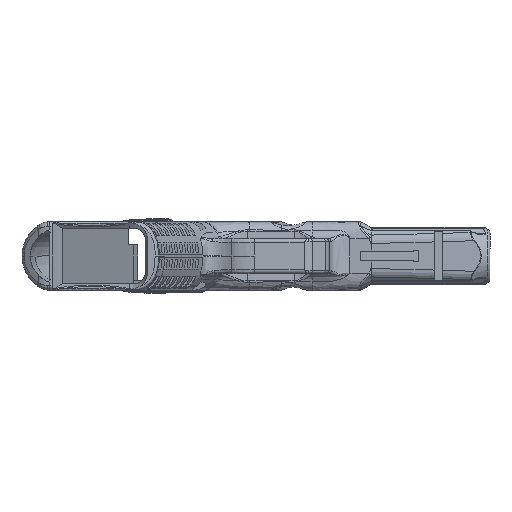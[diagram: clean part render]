
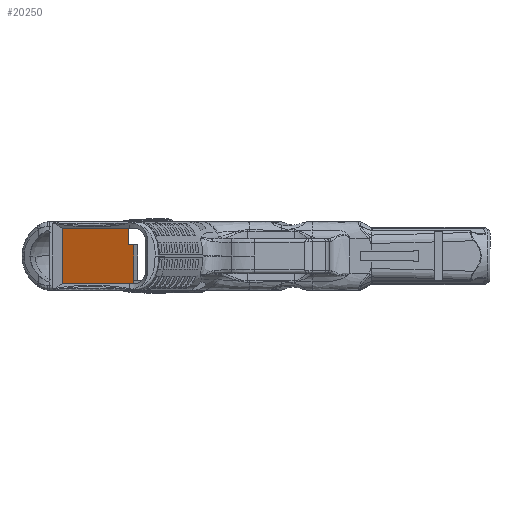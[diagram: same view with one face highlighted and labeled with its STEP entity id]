
A CAD part, front view. The second image highlights one B-rep face of the part: STEP entity #20250.
In plain terms, the highlighted planar face has unit normal (0.95, -0.311, 0).
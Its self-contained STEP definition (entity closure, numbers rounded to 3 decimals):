
#580=PLANE('',#21538);
#2908=FACE_OUTER_BOUND('',#4125,.T.);
#4125=EDGE_LOOP('',(#14632,#14633,#14634,#14635,#14636,#14637,#14638,#14639,
#14640,#14641,#14642));
#5301=LINE('',#34542,#6523);
#5313=LINE('',#35303,#6535);
#5354=LINE('',#42689,#6576);
#5384=LINE('',#45547,#6606);
#5385=LINE('',#45549,#6607);
#5386=LINE('',#45551,#6608);
#5387=LINE('',#45553,#6609);
#5388=LINE('',#45555,#6610);
#5389=LINE('',#45557,#6611);
#5390=LINE('',#45559,#6612);
#5391=LINE('',#45560,#6613);
#6523=VECTOR('',#23052,10.);
#6535=VECTOR('',#23108,10.);
#6576=VECTOR('',#23311,10.);
#6606=VECTOR('',#23455,1.);
#6607=VECTOR('',#23456,10.);
#6608=VECTOR('',#23457,1.);
#6609=VECTOR('',#23458,1.);
#6610=VECTOR('',#23459,1.);
#6611=VECTOR('',#23460,1.);
#6612=VECTOR('',#23461,1.);
#6613=VECTOR('',#23462,1.);
#8376=VERTEX_POINT('',#34539);
#8377=VERTEX_POINT('',#34541);
#8403=VERTEX_POINT('',#35300);
#8404=VERTEX_POINT('',#35302);
#8618=VERTEX_POINT('',#45546);
#8619=VERTEX_POINT('',#45548);
#8620=VERTEX_POINT('',#45550);
#8621=VERTEX_POINT('',#45552);
#8622=VERTEX_POINT('',#45554);
#8623=VERTEX_POINT('',#45556);
#8624=VERTEX_POINT('',#45558);
#10536=EDGE_CURVE('',#8377,#8376,#5301,.T.);
#10577=EDGE_CURVE('',#8403,#8404,#5313,.T.);
#10778=EDGE_CURVE('',#8376,#8404,#5354,.T.);
#10904=EDGE_CURVE('',#8403,#8618,#5384,.T.);
#10905=EDGE_CURVE('',#8618,#8619,#5385,.T.);
#10906=EDGE_CURVE('',#8620,#8619,#5386,.T.);
#10907=EDGE_CURVE('',#8621,#8620,#5387,.T.);
#10908=EDGE_CURVE('',#8621,#8622,#5388,.T.);
#10909=EDGE_CURVE('',#8622,#8623,#5389,.T.);
#10910=EDGE_CURVE('',#8624,#8623,#5390,.T.);
#10911=EDGE_CURVE('',#8377,#8624,#5391,.T.);
#14632=ORIENTED_EDGE('',*,*,#10904,.T.);
#14633=ORIENTED_EDGE('',*,*,#10905,.T.);
#14634=ORIENTED_EDGE('',*,*,#10906,.F.);
#14635=ORIENTED_EDGE('',*,*,#10907,.F.);
#14636=ORIENTED_EDGE('',*,*,#10908,.T.);
#14637=ORIENTED_EDGE('',*,*,#10909,.T.);
#14638=ORIENTED_EDGE('',*,*,#10910,.F.);
#14639=ORIENTED_EDGE('',*,*,#10911,.F.);
#14640=ORIENTED_EDGE('',*,*,#10536,.T.);
#14641=ORIENTED_EDGE('',*,*,#10778,.T.);
#14642=ORIENTED_EDGE('',*,*,#10577,.F.);
#20250=ADVANCED_FACE('',(#2908),#580,.T.);
#21538=AXIS2_PLACEMENT_3D('',#45545,#23453,#23454);
#23052=DIRECTION('',(0.294,0.897,-0.329));
#23108=DIRECTION('',(0.294,0.897,0.329));
#23311=DIRECTION('',(0.,0.,-1.));
#23453=DIRECTION('center_axis',(0.95,-0.311,0.));
#23454=DIRECTION('ref_axis',(0.,0.,
1.));
#23455=DIRECTION('',(0.311,0.95,0.));
#23456=DIRECTION('',(0.,0.,1.));
#23457=DIRECTION('',(0.311,0.95,0.));
#23458=DIRECTION('',(0.311,0.95,0.));
#23459=DIRECTION('',(0.,0.,1.));
#23460=DIRECTION('',(-0.311,-0.95,0.));
#23461=DIRECTION('',(0.,0.,-1.));
#23462=DIRECTION('',(0.311,0.95,0.));
#34539=CARTESIAN_POINT('',(2.433,-97.677,11.632));
#34541=CARTESIAN_POINT('',(2.327,-98.,11.75));
#34542=CARTESIAN_POINT('',(3.562,-94.228,10.367));
#35300=CARTESIAN_POINT('',(2.327,-98.,-11.75));
#35302=CARTESIAN_POINT('',(2.433,-97.677,-11.632));
#35303=CARTESIAN_POINT('',(3.562,-94.228,-10.367));
#42689=CARTESIAN_POINT('',(2.433,-97.677,-18.375));
#45545=CARTESIAN_POINT('Origin',(2.,-99.,-11.75));
#45546=CARTESIAN_POINT('',(32.453,-5.968,-11.75));
#45547=CARTESIAN_POINT('',(2.,-99.,-11.75));
#45548=CARTESIAN_POINT('',(32.453,-5.968,-10.375));
#45549=CARTESIAN_POINT('',(32.453,-5.968,-5.875));
#45550=CARTESIAN_POINT('',(32.448,-5.981,-10.375));
#45551=CARTESIAN_POINT('',(32.119,-6.987,-10.375));
#45552=CARTESIAN_POINT('',(32.448,-5.982,-10.375));
#45553=CARTESIAN_POINT('',(32.119,-6.987,-10.375));
#45554=CARTESIAN_POINT('',(32.448,-5.982,4.75));
#45555=CARTESIAN_POINT('',(32.448,-5.982,-11.75));
#45556=CARTESIAN_POINT('',(30.347,-12.4,4.75));
#45557=CARTESIAN_POINT('',(18.858,-47.499,4.75));
#45558=CARTESIAN_POINT('',(30.347,-12.4,11.75));
#45559=CARTESIAN_POINT('',(30.347,-12.4,2.982));
#45560=CARTESIAN_POINT('',(2.,-99.,11.75));
